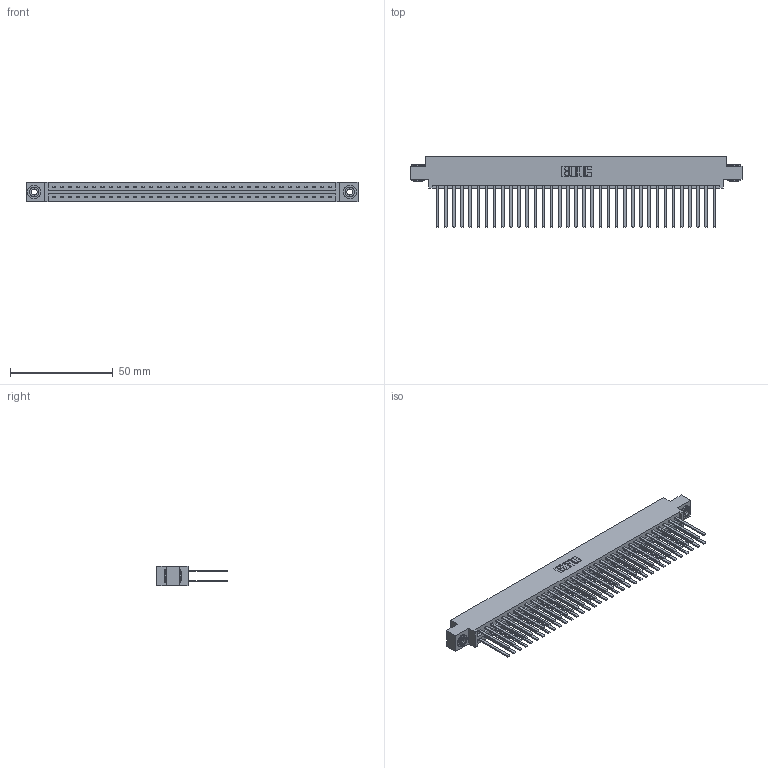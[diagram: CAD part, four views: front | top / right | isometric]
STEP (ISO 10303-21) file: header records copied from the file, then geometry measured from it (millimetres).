
FILE_DESCRIPTION (( 'STEP AP203' ), '1' );
FILE_NAME ('387-070-544-803.STEP', '2019-10-21T22:46:11', ( '' ), ( '' ), 'SwSTEP 2.0', 'SolidWorks 2016', '' );
FILE_SCHEMA (( 'CONFIG_CONTROL_DESIGN' ));
Length unit declared in the file: inch
Products named in the file (4): 345-250-002_345-250-002-102; 387-070-544-803; 337 Part_0.170 Offset - 0.156 Dia-TH; 345-292-001_345-293-144
Assembly tree (73 placements, depth 2):
  387-070-544-803
    337 Part_0.170 Offset - 0.156 Dia-TH
    345-292-001_345-293-144  x70
    345-250-002_345-250-002-102  x2
Bounding box: 161.7 x 34.3 x 9.4 mm (x, y, z)
Volume: 17830.8 mm3; surface area: 23627.6 mm2
Topology: 73 solids, 73 shells, 3516 faces, 10409 edges, 6842 vertices
Faces by surface type: plane 2464, cylinder 1044, cone 8
Entity records: 28640 total; most frequent: CARTESIAN_POINT 4805, ORIENTED_EDGE 4734, DIRECTION 4129, EDGE_CURVE 2367, LINE 2219, VECTOR 2219, VERTEX_POINT 1574, AXIS2_PLACEMENT_3D 955
